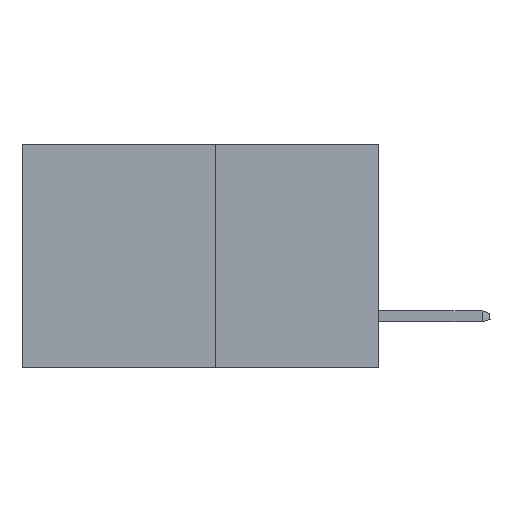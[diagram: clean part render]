
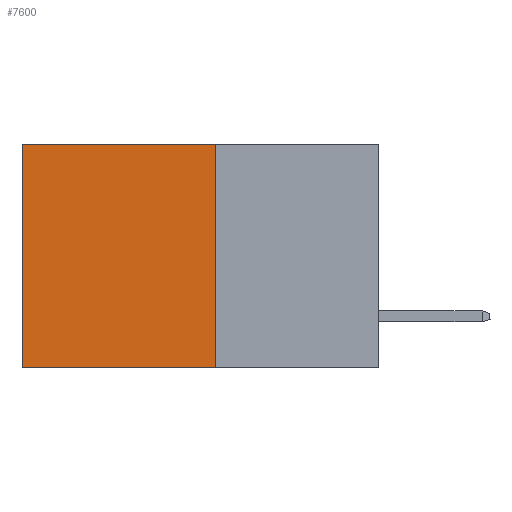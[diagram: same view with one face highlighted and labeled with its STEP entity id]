
A CAD part, left-side view. The second image highlights one B-rep face of the part: STEP entity #7600.
In plain terms, the highlighted planar face has unit normal (-1, 0, 0).
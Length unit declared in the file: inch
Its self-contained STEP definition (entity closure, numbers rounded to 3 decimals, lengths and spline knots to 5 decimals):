
#1187 = DIRECTION ( 'NONE',  ( 0., 1., 0. ) ) ;
#1672 = ORIENTED_EDGE ( 'NONE', *, *, #21927, .T. ) ;
#3687 = LINE ( 'NONE', #8931, #29521 ) ;
#5460 = EDGE_CURVE ( 'NONE', #22872, #27957, #14097, .T. ) ;
#5560 = DIRECTION ( 'NONE',  ( 1., 0., 0. ) ) ;
#6138 = CARTESIAN_POINT ( 'NONE',  ( 0.277, 0.27, -0.37 ) ) ;
#7363 = ORIENTED_EDGE ( 'NONE', *, *, #5460, .T. ) ;
#7600 = ADVANCED_FACE ( 'NONE', ( #32099 ), #15707, .F. ) ;
#8931 = CARTESIAN_POINT ( 'NONE',  ( 0.277, 0.27, 0. ) ) ;
#10111 = CARTESIAN_POINT ( 'NONE',  ( 0.277, 0.27, -0.37 ) ) ;
#11583 = LINE ( 'NONE', #10111, #25712 ) ;
#11709 = CARTESIAN_POINT ( 'NONE',  ( 0.277, 0.59, -0.37 ) ) ;
#12028 = LINE ( 'NONE', #6138, #24588 ) ;
#14086 = DIRECTION ( 'NONE',  ( 0., 1., 0. ) ) ;
#14097 = LINE ( 'NONE', #11709, #20023 ) ;
#15596 = CARTESIAN_POINT ( 'NONE',  ( 0.277, 0.59, -0.37 ) ) ;
#15707 = PLANE ( 'NONE',  #22160 ) ;
#15847 = ORIENTED_EDGE ( 'NONE', *, *, #22565, .F. ) ;
#16101 = EDGE_LOOP ( 'NONE', ( #7363, #15847, #29148, #1672 ) ) ;
#16265 = EDGE_CURVE ( 'NONE', #31943, #24004, #11583, .T. ) ;
#18913 = CARTESIAN_POINT ( 'NONE',  ( 0.277, 0.27, 0. ) ) ;
#19855 = CARTESIAN_POINT ( 'NONE',  ( 0.277, 0.27, -0.37 ) ) ;
#20023 = VECTOR ( 'NONE', #31574, 39.37008 ) ;
#20730 = CARTESIAN_POINT ( 'NONE',  ( 0.277, 0.27, -0.37 ) ) ;
#21927 = EDGE_CURVE ( 'NONE', #31943, #22872, #3687, .T. ) ;
#22160 = AXIS2_PLACEMENT_3D ( 'NONE', #20730, #5560, #23225 ) ;
#22565 = EDGE_CURVE ( 'NONE', #24004, #27957, #12028, .T. ) ;
#22710 = DIRECTION ( 'NONE',  ( 0., 0., -1. ) ) ;
#22872 = VERTEX_POINT ( 'NONE', #32102 ) ;
#23225 = DIRECTION ( 'NONE',  ( 0., 0., -1. ) ) ;
#24004 = VERTEX_POINT ( 'NONE', #19855 ) ;
#24588 = VECTOR ( 'NONE', #1187, 39.37008 ) ;
#25712 = VECTOR ( 'NONE', #22710, 39.37008 ) ;
#27957 = VERTEX_POINT ( 'NONE', #15596 ) ;
#29148 = ORIENTED_EDGE ( 'NONE', *, *, #16265, .F. ) ;
#29521 = VECTOR ( 'NONE', #14086, 39.37008 ) ;
#31574 = DIRECTION ( 'NONE',  ( 0., 0., -1. ) ) ;
#31943 = VERTEX_POINT ( 'NONE', #18913 ) ;
#32099 = FACE_OUTER_BOUND ( 'NONE', #16101, .T. ) ;
#32102 = CARTESIAN_POINT ( 'NONE',  ( 0.277, 0.59, 0. ) ) ;
